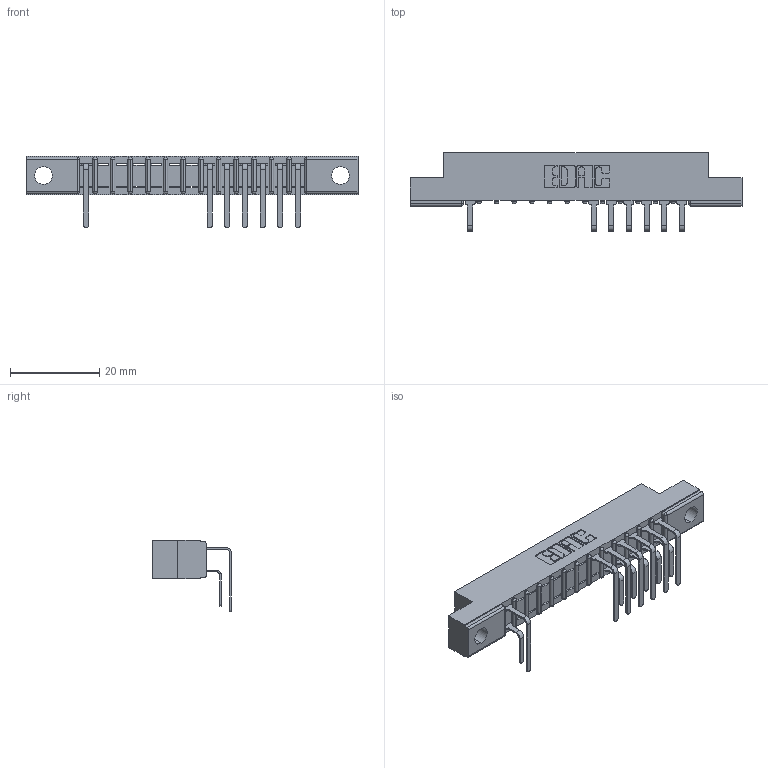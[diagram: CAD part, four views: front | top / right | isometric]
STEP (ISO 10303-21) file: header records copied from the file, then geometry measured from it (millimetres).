
FILE_DESCRIPTION (( 'STEP AP203' ), '1' );
FILE_NAME ('307-026-559-202.STEP', '2018-08-04T14:43:27', ( '' ), ( '' ), 'SwSTEP 2.0', 'SolidWorks 2016', '' );
FILE_SCHEMA (( 'CONFIG_CONTROL_DESIGN' ));
Length unit declared in the file: inch
Products named in the file (4): 307-290-001_558 559 - 1 (Single); 307-290-001_559 - 2 (Single); 307-026-559-202; 307 Part_.128 Dia Mounting Holes
Assembly tree (14 placements, depth 2):
  307-026-559-202
    307 Part_.128 Dia Mounting Holes
    307-290-001_558 559 - 1 (Single)  x6
    307-290-001_559 - 2 (Single)  x7
Bounding box: 74.52 x 17.69 x 16.08 mm (x, y, z)
Volume: 4678.8 mm3; surface area: 6981.7 mm2
Topology: 14 solids, 14 shells, 912 faces, 2585 edges, 1666 vertices
Faces by surface type: plane 577, cylinder 307, sphere 28
Entity records: 16169 total; most frequent: CARTESIAN_POINT 2710, ORIENTED_EDGE 2694, DIRECTION 2653, EDGE_CURVE 1347, VECTOR 1019, LINE 1019, VERTEX_POINT 874, AXIS2_PLACEMENT_3D 817
